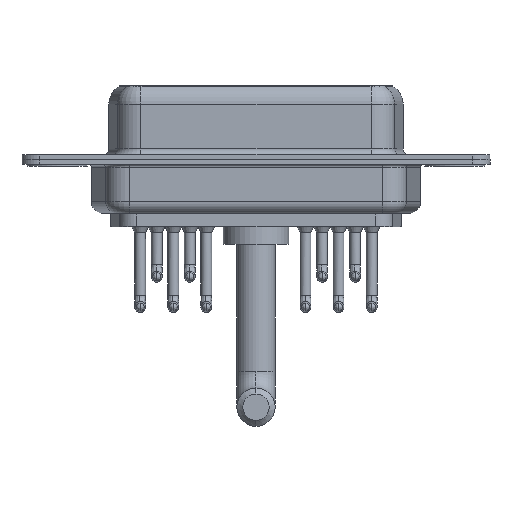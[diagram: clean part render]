
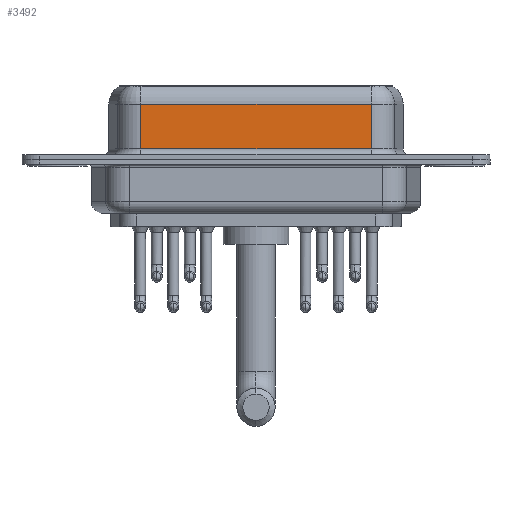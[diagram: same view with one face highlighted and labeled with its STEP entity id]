
A CAD part, front view. The second image highlights one B-rep face of the part: STEP entity #3492.
In plain terms, the highlighted planar face has unit normal (0, -1, 0).
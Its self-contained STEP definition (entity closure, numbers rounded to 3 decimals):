
#1065 = LINE ( 'NONE', #2344, #6072 ) ;
#1579 = EDGE_CURVE ( 'NONE', #10398, #7802, #9823, .T. ) ;
#2344 = CARTESIAN_POINT ( 'NONE',  ( 26.287, -3.95, 0.9 ) ) ;
#2540 = CARTESIAN_POINT ( 'NONE',  ( 7.013, -3.95, 4.65 ) ) ;
#2578 = EDGE_CURVE ( 'NONE', #16712, #7802, #1065, .T. ) ;
#2782 = DIRECTION ( 'NONE',  ( 0., 0., -1. ) ) ;
#2851 = CARTESIAN_POINT ( 'NONE',  ( 26.287, -3.95, 0.9 ) ) ;
#2993 = CARTESIAN_POINT ( 'NONE',  ( 26.287, -3.95, 6.4 ) ) ;
#3492 = ADVANCED_FACE ( 'NONE', ( #12534 ), #7591, .F. ) ;
#3845 = VECTOR ( 'NONE', #16144, 1000. ) ;
#5391 = VECTOR ( 'NONE', #16115, 1000. ) ;
#5529 = VERTEX_POINT ( 'NONE', #2540 ) ;
#6072 = VECTOR ( 'NONE', #15234, 1000. ) ;
#6217 = ORIENTED_EDGE ( 'NONE', *, *, #12462, .T. ) ;
#6373 = AXIS2_PLACEMENT_3D ( 'NONE', #9979, #16625, #16458 ) ;
#7591 = PLANE ( 'NONE',  #6373 ) ;
#7802 = VERTEX_POINT ( 'NONE', #2851 ) ;
#8181 = CARTESIAN_POINT ( 'NONE',  ( 26.287, -3.95, 4.65 ) ) ;
#8256 = EDGE_LOOP ( 'NONE', ( #8472, #6217, #15986, #8964 ) ) ;
#8472 = ORIENTED_EDGE ( 'NONE', *, *, #1579, .F. ) ;
#8964 = ORIENTED_EDGE ( 'NONE', *, *, #2578, .T. ) ;
#9383 = LINE ( 'NONE', #8181, #5391 ) ;
#9823 = LINE ( 'NONE', #2993, #3845 ) ;
#9979 = CARTESIAN_POINT ( 'NONE',  ( 26.287, -3.95, 6.4 ) ) ;
#10398 = VERTEX_POINT ( 'NONE', #12730 ) ;
#12462 = EDGE_CURVE ( 'NONE', #10398, #5529, #9383, .T. ) ;
#12534 = FACE_OUTER_BOUND ( 'NONE', #8256, .T. ) ;
#12730 = CARTESIAN_POINT ( 'NONE',  ( 26.287, -3.95, 4.65 ) ) ;
#12941 = LINE ( 'NONE', #15587, #13904 ) ;
#13904 = VECTOR ( 'NONE', #2782, 1000. ) ;
#14974 = EDGE_CURVE ( 'NONE', #5529, #16712, #12941, .T. ) ;
#15234 = DIRECTION ( 'NONE',  ( 1., 0., 0. ) ) ;
#15587 = CARTESIAN_POINT ( 'NONE',  ( 7.013, -3.95, 6.4 ) ) ;
#15986 = ORIENTED_EDGE ( 'NONE', *, *, #14974, .T. ) ;
#16115 = DIRECTION ( 'NONE',  ( -1., 0., 0. ) ) ;
#16144 = DIRECTION ( 'NONE',  ( 0., 0., -1. ) ) ;
#16458 = DIRECTION ( 'NONE',  ( 0., 0., 1. ) ) ;
#16625 = DIRECTION ( 'NONE',  ( 0., 1., 0. ) ) ;
#16706 = CARTESIAN_POINT ( 'NONE',  ( 7.013, -3.95, 0.9 ) ) ;
#16712 = VERTEX_POINT ( 'NONE', #16706 ) ;
